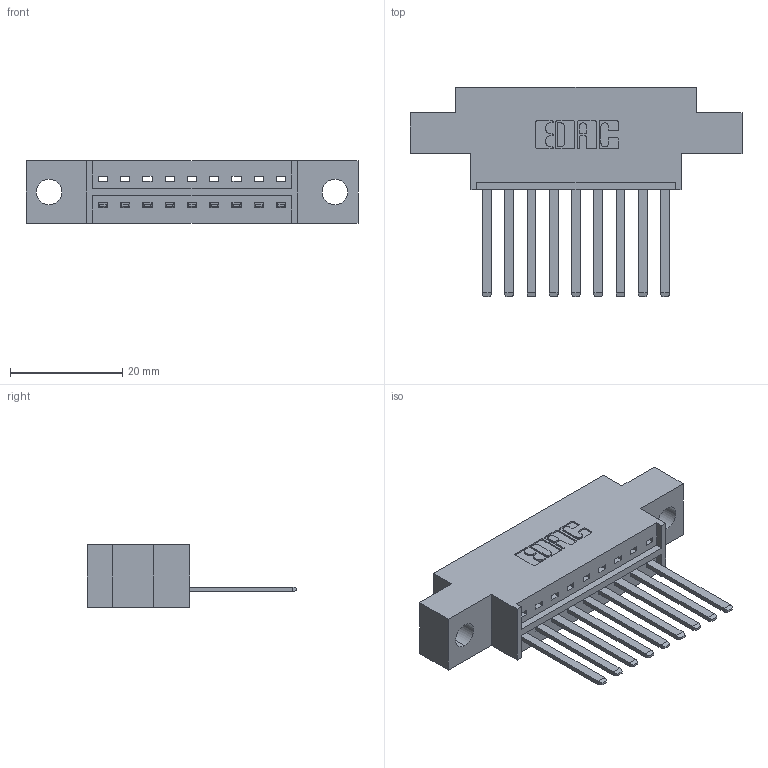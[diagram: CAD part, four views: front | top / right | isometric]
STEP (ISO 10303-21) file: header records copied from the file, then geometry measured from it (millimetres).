
FILE_DESCRIPTION (( 'STEP AP203' ), '1' );
FILE_NAME ('336-009-541-609.STEP', '2020-08-07T19:28:03', ( '' ), ( '' ), 'SwSTEP 2.0', 'SolidWorks 2020', '' );
FILE_SCHEMA (( 'CONFIG_CONTROL_DESIGN' ));
Length unit declared in the file: inch
Products named in the file (3): 336-009-541-609; 336 Part_Offset - .178 Dia - TH; 336-290-001_336-290-541
Assembly tree (10 placements, depth 2):
  336-009-541-609
    336 Part_Offset - .178 Dia - TH
    336-290-001_336-290-541  x9
Bounding box: 59.05 x 37.34 x 11.1 mm (x, y, z)
Volume: 7508.3 mm3; surface area: 7700.4 mm2
Topology: 10 solids, 10 shells, 568 faces, 1709 edges, 1132 vertices
Faces by surface type: plane 380, cylinder 188
Entity records: 10812 total; most frequent: CARTESIAN_POINT 1972, ORIENTED_EDGE 1818, DIRECTION 1631, EDGE_CURVE 909, VECTOR 777, LINE 777, VERTEX_POINT 604, AXIS2_PLACEMENT_3D 427
